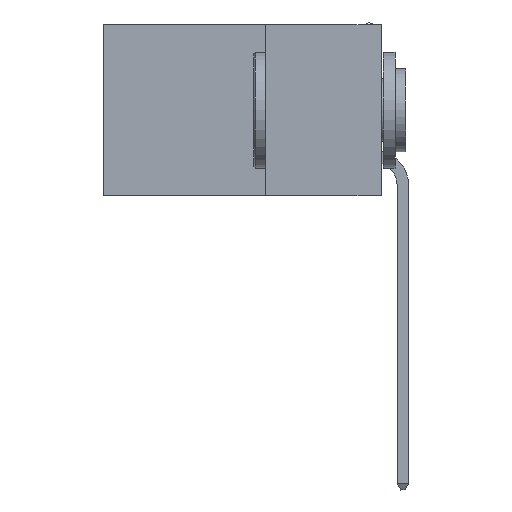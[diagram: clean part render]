
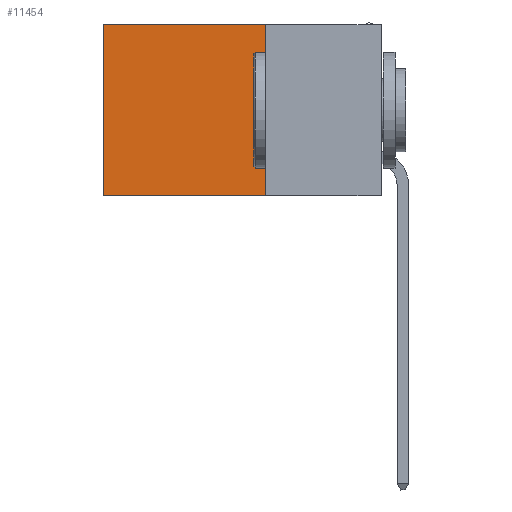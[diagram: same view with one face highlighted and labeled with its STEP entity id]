
A CAD part, left-side view. The second image highlights one B-rep face of the part: STEP entity #11454.
In plain terms, the highlighted planar face has unit normal (-1, 0, 0).
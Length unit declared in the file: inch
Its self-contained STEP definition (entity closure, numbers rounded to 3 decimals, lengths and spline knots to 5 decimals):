
#846 = ORIENTED_EDGE ( 'NONE', *, *, #14387, .F. ) ;
#1521 = DIRECTION ( 'NONE',  ( 0., 1., 0. ) ) ;
#1878 = VERTEX_POINT ( 'NONE', #13018 ) ;
#2229 = DIRECTION ( 'NONE',  ( 0., 0., -1. ) ) ;
#2797 = CARTESIAN_POINT ( 'NONE',  ( 0.2875, 0.25, -0.37 ) ) ;
#2818 = EDGE_CURVE ( 'NONE', #11286, #1878, #4817, .T. ) ;
#3238 = VECTOR ( 'NONE', #1521, 39.37008 ) ;
#4092 = CARTESIAN_POINT ( 'NONE',  ( 0.2875, 0.25, -0.37 ) ) ;
#4142 = PLANE ( 'NONE',  #5607 ) ;
#4817 = LINE ( 'NONE', #12765, #14369 ) ;
#5404 = DIRECTION ( 'NONE',  ( 0., 0., -1. ) ) ;
#5607 = AXIS2_PLACEMENT_3D ( 'NONE', #7924, #12882, #5404 ) ;
#6816 = EDGE_CURVE ( 'NONE', #9600, #11286, #12107, .T. ) ;
#7753 = EDGE_LOOP ( 'NONE', ( #8910, #9119, #846, #15099 ) ) ;
#7924 = CARTESIAN_POINT ( 'NONE',  ( 0.2875, 0.25, 0. ) ) ;
#8538 = VECTOR ( 'NONE', #2229, 39.37008 ) ;
#8910 = ORIENTED_EDGE ( 'NONE', *, *, #2818, .T. ) ;
#8930 = LINE ( 'NONE', #9768, #8538 ) ;
#8946 = FACE_OUTER_BOUND ( 'NONE', #7753, .T. ) ;
#9119 = ORIENTED_EDGE ( 'NONE', *, *, #10723, .F. ) ;
#9600 = VERTEX_POINT ( 'NONE', #10128 ) ;
#9768 = CARTESIAN_POINT ( 'NONE',  ( 0.2875, 0.25, 0. ) ) ;
#9918 = LINE ( 'NONE', #2797, #3238 ) ;
#10128 = CARTESIAN_POINT ( 'NONE',  ( 0.2875, 0.25, 0. ) ) ;
#10250 = VECTOR ( 'NONE', #10307, 39.37008 ) ;
#10307 = DIRECTION ( 'NONE',  ( 0., 1., 0. ) ) ;
#10723 = EDGE_CURVE ( 'NONE', #13220, #1878, #9918, .T. ) ;
#11286 = VERTEX_POINT ( 'NONE', #16229 ) ;
#11454 = ADVANCED_FACE ( 'NONE', ( #8946 ), #4142, .F. ) ;
#12107 = LINE ( 'NONE', #15246, #10250 ) ;
#12335 = DIRECTION ( 'NONE',  ( 0., 0., -1. ) ) ;
#12765 = CARTESIAN_POINT ( 'NONE',  ( 0.2875, 0.6, 0. ) ) ;
#12882 = DIRECTION ( 'NONE',  ( 1., 0., 0. ) ) ;
#13018 = CARTESIAN_POINT ( 'NONE',  ( 0.2875, 0.6, -0.37 ) ) ;
#13220 = VERTEX_POINT ( 'NONE', #4092 ) ;
#14369 = VECTOR ( 'NONE', #12335, 39.37008 ) ;
#14387 = EDGE_CURVE ( 'NONE', #9600, #13220, #8930, .T. ) ;
#15099 = ORIENTED_EDGE ( 'NONE', *, *, #6816, .T. ) ;
#15246 = CARTESIAN_POINT ( 'NONE',  ( 0.2875, 0.25, 0. ) ) ;
#16229 = CARTESIAN_POINT ( 'NONE',  ( 0.2875, 0.6, 0. ) ) ;
